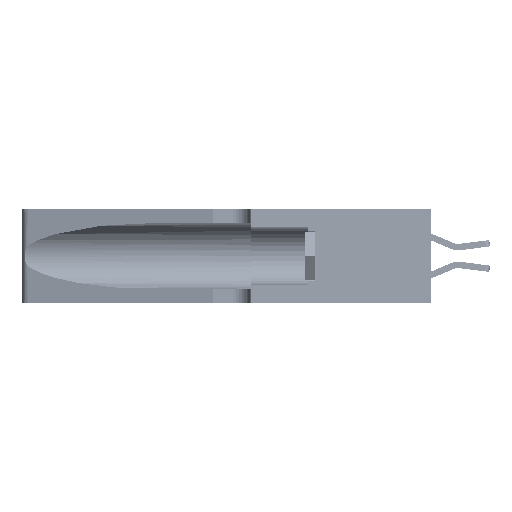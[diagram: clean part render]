
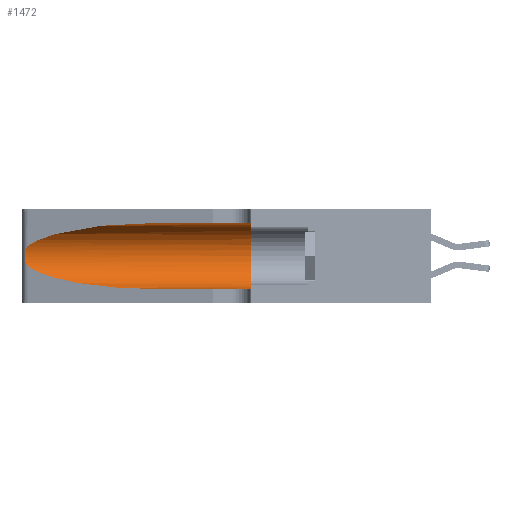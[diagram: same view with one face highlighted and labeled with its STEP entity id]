
A CAD part, left-side view. The second image highlights one B-rep face of the part: STEP entity #1472.
In plain terms, the highlighted cylindrical face has radius 3.308 mm (diameter 6.617 mm), a partial arc.
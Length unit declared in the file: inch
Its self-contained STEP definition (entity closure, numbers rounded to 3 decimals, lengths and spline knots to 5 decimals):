
#498 = CARTESIAN_POINT ( 'NONE',  ( 0.25789, 1.23486, 0.15765 ) ) ;
#808 = CARTESIAN_POINT ( 'NONE',  ( 0.1305, 0.35, 0.05475 ) ) ;
#1382 = CARTESIAN_POINT ( 'NONE',  ( 0.25854, 1.2359, 0.20912 ) ) ;
#1455 = CARTESIAN_POINT ( 'NONE',  ( 0.1305, 1.61858, 0.185 ) ) ;
#1472 = ADVANCED_FACE ( 'NONE', ( #15732 ), #6048, .F. ) ;
#1678 = DIRECTION ( 'NONE',  ( 0., 1., 0. ) ) ;
#2851 = AXIS2_PLACEMENT_3D ( 'NONE', #14746, #1678, #21357 ) ;
#2975 = CARTESIAN_POINT ( 'NONE',  ( 0.18966, 0.96281, 0.05475 ) ) ;
#3775 = CARTESIAN_POINT ( 'NONE',  ( 0.25487, 1.22718, 0.22369 ) ) ;
#3945 = CIRCLE ( 'NONE', #2851, 0.13025 ) ;
#4664 = AXIS2_PLACEMENT_3D ( 'NONE', #1455, #15187, #8147 ) ;
#5297 = CARTESIAN_POINT ( 'NONE',  ( 0.25487, 1.22718, 0.22369 ) ) ;
#5646 = DIRECTION ( 'NONE',  ( 0., -1., 0. ) ) ;
#6048 = CYLINDRICAL_SURFACE ( 'NONE', #4664, 0.13025 ) ;
#6387 = CARTESIAN_POINT ( 'NONE',  ( 0.25487, 1.22718, 0.14631 ) ) ;
#6465 = ORIENTED_EDGE ( 'NONE', *, *, #23641, .T. ) ;
#6549 = VECTOR ( 'NONE', #5646, 39.37008 ) ;
#7002 = LINE ( 'NONE', #8750, #6549 ) ;
#7596 = CARTESIAN_POINT ( 'NONE',  ( 0.26018, 1.23835, 0.19895 ) ) ;
#8147 = DIRECTION ( 'NONE',  ( 0., 0., -1. ) ) ;
#8750 = CARTESIAN_POINT ( 'NONE',  ( 0.1305, 1.61858, 0.05475 ) ) ;
#8944 = CARTESIAN_POINT ( 'NONE',  ( 0.25487, 1.22718, 0.22369 ) ) ;
#9150 = CARTESIAN_POINT ( 'NONE',  ( 0.25555, 1.22993, 0.14849 ) ) ;
#9428 = VERTEX_POINT ( 'NONE', #5297 ) ;
#11675 = CARTESIAN_POINT ( 'NONE',  ( 0.25856, 1.23593, 0.16098 ) ) ;
#12010 = EDGE_CURVE ( 'NONE', #39958, #40970, #25315, .T. ) ;
#13049 = EDGE_CURVE ( 'NONE', #19358, #9428, #35212, .T. ) ;
#13409 = EDGE_CURVE ( 'NONE', #19358, #18892, #31849, .T. ) ;
#14656 = CARTESIAN_POINT ( 'NONE',  ( 0.2373, 1.15595, 0.28018 ) ) ;
#14746 = CARTESIAN_POINT ( 'NONE',  ( 0.1305, 0.35, 0.185 ) ) ;
#15187 = DIRECTION ( 'NONE',  ( 0., -1., 0. ) ) ;
#15732 = FACE_OUTER_BOUND ( 'NONE', #28414, .T. ) ;
#16035 = CARTESIAN_POINT ( 'NONE',  ( 0.1305, 0.72297, 0.05475 ) ) ;
#16447 = EDGE_CURVE ( 'NONE', #18892, #21999, #3945, .T. ) ;
#16869 = CARTESIAN_POINT ( 'NONE',  ( 0.25555, 1.22994, 0.2215 ) ) ;
#17548 = CARTESIAN_POINT ( 'NONE',  ( 0.25487, 1.22718, 0.14631 ) ) ;
#18892 = VERTEX_POINT ( 'NONE', #27156 ) ;
#19358 = VERTEX_POINT ( 'NONE', #23835 ) ;
#20464 = CARTESIAN_POINT ( 'NONE',  ( 0.25487, 1.22718, 0.14631 ) ) ;
#21063 = CARTESIAN_POINT ( 'NONE',  ( 0.25639, 1.23184, 0.21858 ) ) ;
#21357 = DIRECTION ( 'NONE',  ( 0., 0., 1. ) ) ;
#21999 = VERTEX_POINT ( 'NONE', #808 ) ;
#22391 = CARTESIAN_POINT ( 'NONE',  ( 0.1305, 1.61858, 0.31525 ) ) ;
#22511 = CARTESIAN_POINT ( 'NONE',  ( 0.2373, 1.15595, 0.08982 ) ) ;
#23641 = EDGE_CURVE ( 'NONE', #9428, #39958, #28447, .T. ) ;
#23835 = CARTESIAN_POINT ( 'NONE',  ( 0.1305, 0.72297, 0.31525 ) ) ;
#24400 = CARTESIAN_POINT ( 'NONE',  ( 0.18966, 0.96281, 0.31525 ) ) ;
#25315 =( BOUNDED_CURVE ( )  B_SPLINE_CURVE ( 3, ( #20464, #22511, #2975, #36266 ),
 .UNSPECIFIED., .F., .F. ) 
 B_SPLINE_CURVE_WITH_KNOTS ( ( 4, 4 ),
 ( 3.44316, 4.71239 ),
 .UNSPECIFIED. ) 
 CURVE ( )  GEOMETRIC_REPRESENTATION_ITEM ( )  RATIONAL_B_SPLINE_CURVE ( ( 1., 0.87, 0.87, 1. ) ) 
 REPRESENTATION_ITEM ( '' )  );
#26190 = VECTOR ( 'NONE', #29216, 39.37008 ) ;
#27156 = CARTESIAN_POINT ( 'NONE',  ( 0.1305, 0.35, 0.31525 ) ) ;
#28414 = EDGE_LOOP ( 'NONE', ( #38044, #6465, #37575, #31512, #29992, #39041 ) ) ;
#28447 = B_SPLINE_CURVE_WITH_KNOTS ( 'NONE', 3,
 ( #3775, #16869, #21063, #40068, #1382, #7596, #33705, #35523, #33500, #11675, #498, #31088, #9150, #6387 ),
 .UNSPECIFIED., .F., .F.,
 ( 4, 2, 2, 2, 2, 2, 4 ),
 ( 0., 0.00027, 0.00053, 0.00107, 0.0016, 0.00187, 0.00214 ),
 .UNSPECIFIED. ) ;
#29216 = DIRECTION ( 'NONE',  ( 0., -1., 0. ) ) ;
#29992 = ORIENTED_EDGE ( 'NONE', *, *, #16447, .F. ) ;
#30829 = CARTESIAN_POINT ( 'NONE',  ( 0.1305, 0.72297, 0.31525 ) ) ;
#31088 = CARTESIAN_POINT ( 'NONE',  ( 0.25639, 1.23186, 0.15144 ) ) ;
#31512 = ORIENTED_EDGE ( 'NONE', *, *, #38933, .T. ) ;
#31849 = LINE ( 'NONE', #22391, #26190 ) ;
#33500 = CARTESIAN_POINT ( 'NONE',  ( 0.26017, 1.23833, 0.17102 ) ) ;
#33705 = CARTESIAN_POINT ( 'NONE',  ( 0.26075, 1.23896, 0.19203 ) ) ;
#35212 =( BOUNDED_CURVE ( )  B_SPLINE_CURVE ( 3, ( #30829, #24400, #14656, #8944 ),
 .UNSPECIFIED., .F., .T. ) 
 B_SPLINE_CURVE_WITH_KNOTS ( ( 4, 4 ),
 ( 1.5708, 2.84003 ),
 .UNSPECIFIED. ) 
 CURVE ( )  GEOMETRIC_REPRESENTATION_ITEM ( )  RATIONAL_B_SPLINE_CURVE ( ( 1., 0.87, 0.87, 1. ) ) 
 REPRESENTATION_ITEM ( '' )  );
#35523 = CARTESIAN_POINT ( 'NONE',  ( 0.26075, 1.23896, 0.178 ) ) ;
#36266 = CARTESIAN_POINT ( 'NONE',  ( 0.1305, 0.72297, 0.05475 ) ) ;
#37575 = ORIENTED_EDGE ( 'NONE', *, *, #12010, .T. ) ;
#38044 = ORIENTED_EDGE ( 'NONE', *, *, #13049, .T. ) ;
#38933 = EDGE_CURVE ( 'NONE', #40970, #21999, #7002, .T. ) ;
#39041 = ORIENTED_EDGE ( 'NONE', *, *, #13409, .F. ) ;
#39958 = VERTEX_POINT ( 'NONE', #17548 ) ;
#40068 = CARTESIAN_POINT ( 'NONE',  ( 0.25787, 1.23484, 0.2124 ) ) ;
#40970 = VERTEX_POINT ( 'NONE', #16035 ) ;
